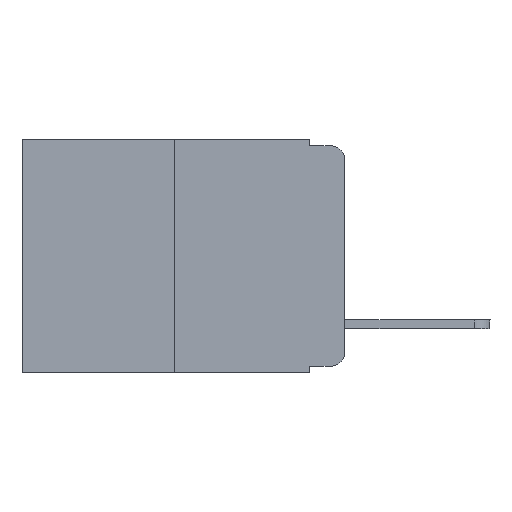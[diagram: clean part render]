
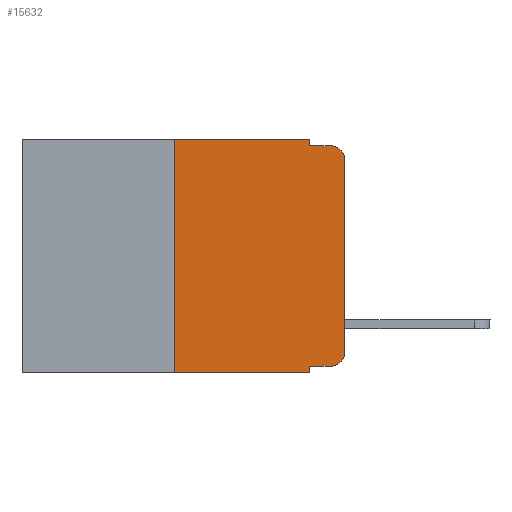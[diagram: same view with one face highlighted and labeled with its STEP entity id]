
A CAD part, left-side view. The second image highlights one B-rep face of the part: STEP entity #15632.
In plain terms, the highlighted planar face has unit normal (-1, 0, 0).
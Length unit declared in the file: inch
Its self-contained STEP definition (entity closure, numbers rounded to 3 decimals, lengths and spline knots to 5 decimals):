
#16 = VERTEX_POINT ( 'NONE', #12961 ) ;
#89 = ORIENTED_EDGE ( 'NONE', *, *, #2697, .T. ) ;
#447 = LINE ( 'NONE', #6136, #10270 ) ;
#598 = VECTOR ( 'NONE', #6425, 39.37008 ) ;
#610 = DIRECTION ( 'NONE',  ( 0., -1., 0. ) ) ;
#771 = EDGE_CURVE ( 'NONE', #15232, #12981, #5989, .T. ) ;
#961 = EDGE_CURVE ( 'NONE', #3831, #3581, #9354, .T. ) ;
#1039 = CARTESIAN_POINT ( 'NONE',  ( 0., 0.25, 0. ) ) ;
#1077 = VERTEX_POINT ( 'NONE', #1764 ) ;
#1095 = DIRECTION ( 'NONE',  ( 0., 0., 1. ) ) ;
#1254 = EDGE_CURVE ( 'NONE', #3831, #16, #9566, .T. ) ;
#1634 = DIRECTION ( 'NONE',  ( -1., 0., 0. ) ) ;
#1764 = CARTESIAN_POINT ( 'NONE',  ( 0., 0.051, 0. ) ) ;
#2280 = AXIS2_PLACEMENT_3D ( 'NONE', #14104, #15398, #8887 ) ;
#2580 = VERTEX_POINT ( 'NONE', #16187 ) ;
#2617 = ORIENTED_EDGE ( 'NONE', *, *, #11180, .T. ) ;
#2697 = EDGE_CURVE ( 'NONE', #2580, #15232, #8344, .T. ) ;
#2749 = CARTESIAN_POINT ( 'NONE',  ( 0., 0.02, -0.313 ) ) ;
#2760 = EDGE_CURVE ( 'NONE', #16, #1077, #10550, .T. ) ;
#3581 = VERTEX_POINT ( 'NONE', #16235 ) ;
#3825 = ORIENTED_EDGE ( 'NONE', *, *, #13340, .F. ) ;
#3831 = VERTEX_POINT ( 'NONE', #13111 ) ;
#3943 = DIRECTION ( 'NONE',  ( 0., 0., -1. ) ) ;
#3953 = VECTOR ( 'NONE', #12340, 39.37008 ) ;
#4468 = EDGE_LOOP ( 'NONE', ( #5801, #16324, #7175, #3825, #14455, #10237, #12030, #13215, #2617, #89 ) ) ;
#5530 = VECTOR ( 'NONE', #5571, 39.37008 ) ;
#5571 = DIRECTION ( 'NONE',  ( 0., -1., 0. ) ) ;
#5767 = EDGE_CURVE ( 'NONE', #12981, #6544, #14261, .T. ) ;
#5786 = CARTESIAN_POINT ( 'NONE',  ( 0., 0., 0. ) ) ;
#5801 = ORIENTED_EDGE ( 'NONE', *, *, #771, .T. ) ;
#5950 = VERTEX_POINT ( 'NONE', #6956 ) ;
#5989 = LINE ( 'NONE', #5786, #3953 ) ;
#6136 = CARTESIAN_POINT ( 'NONE',  ( 0., 0.051, -0.01 ) ) ;
#6361 = FACE_OUTER_BOUND ( 'NONE', #4468, .T. ) ;
#6425 = DIRECTION ( 'NONE',  ( 0., 0., -1. ) ) ;
#6487 = VECTOR ( 'NONE', #610, 39.37008 ) ;
#6544 = VERTEX_POINT ( 'NONE', #12249 ) ;
#6956 = CARTESIAN_POINT ( 'NONE',  ( 0., 0.051, -0.01 ) ) ;
#7154 = VECTOR ( 'NONE', #1095, 39.37008 ) ;
#7175 = ORIENTED_EDGE ( 'NONE', *, *, #12117, .F. ) ;
#7408 = LINE ( 'NONE', #12821, #598 ) ;
#7543 = LINE ( 'NONE', #7878, #11759 ) ;
#7745 = CARTESIAN_POINT ( 'NONE',  ( 0., 0.051, -0.333 ) ) ;
#7878 = CARTESIAN_POINT ( 'NONE',  ( 0., 0.051, 0. ) ) ;
#8079 = CARTESIAN_POINT ( 'NONE',  ( 0., 0.02, -0.03 ) ) ;
#8344 = CIRCLE ( 'NONE', #10968, 0.02 ) ;
#8750 = DIRECTION ( 'NONE',  ( 0., -1., 0. ) ) ;
#8887 = DIRECTION ( 'NONE',  ( 0., 0., -1. ) ) ;
#8998 = DIRECTION ( 'NONE',  ( -1., 0., 0. ) ) ;
#9354 = LINE ( 'NONE', #15465, #11767 ) ;
#9566 = LINE ( 'NONE', #1039, #7154 ) ;
#10237 = ORIENTED_EDGE ( 'NONE', *, *, #1254, .F. ) ;
#10270 = VECTOR ( 'NONE', #8750, 39.37008 ) ;
#10550 = LINE ( 'NONE', #15828, #5530 ) ;
#10968 = AXIS2_PLACEMENT_3D ( 'NONE', #2749, #8998, #11794 ) ;
#11180 = EDGE_CURVE ( 'NONE', #12218, #2580, #11292, .T. ) ;
#11292 = LINE ( 'NONE', #14674, #6487 ) ;
#11759 = VECTOR ( 'NONE', #3943, 39.37008 ) ;
#11767 = VECTOR ( 'NONE', #14229, 39.37008 ) ;
#11794 = DIRECTION ( 'NONE',  ( 0., 0., -1. ) ) ;
#11933 = DIRECTION ( 'NONE',  ( 0., 0., -1. ) ) ;
#12030 = ORIENTED_EDGE ( 'NONE', *, *, #961, .T. ) ;
#12117 = EDGE_CURVE ( 'NONE', #5950, #6544, #447, .T. ) ;
#12218 = VERTEX_POINT ( 'NONE', #7745 ) ;
#12249 = CARTESIAN_POINT ( 'NONE',  ( 0., 0.02, -0.01 ) ) ;
#12340 = DIRECTION ( 'NONE',  ( 0., 0., 1. ) ) ;
#12603 = AXIS2_PLACEMENT_3D ( 'NONE', #8079, #1634, #11933 ) ;
#12821 = CARTESIAN_POINT ( 'NONE',  ( 0., 0.051, 0. ) ) ;
#12961 = CARTESIAN_POINT ( 'NONE',  ( 0., 0.25, 0. ) ) ;
#12981 = VERTEX_POINT ( 'NONE', #16070 ) ;
#13111 = CARTESIAN_POINT ( 'NONE',  ( 0., 0.25, -0.343 ) ) ;
#13215 = ORIENTED_EDGE ( 'NONE', *, *, #15668, .F. ) ;
#13340 = EDGE_CURVE ( 'NONE', #1077, #5950, #7408, .T. ) ;
#14104 = CARTESIAN_POINT ( 'NONE',  ( 0., 0.473, 0. ) ) ;
#14229 = DIRECTION ( 'NONE',  ( 0., -1., 0. ) ) ;
#14261 = CIRCLE ( 'NONE', #12603, 0.02 ) ;
#14455 = ORIENTED_EDGE ( 'NONE', *, *, #2760, .F. ) ;
#14674 = CARTESIAN_POINT ( 'NONE',  ( 0., 0.051, -0.333 ) ) ;
#15232 = VERTEX_POINT ( 'NONE', #15687 ) ;
#15398 = DIRECTION ( 'NONE',  ( 1., 0., 0. ) ) ;
#15465 = CARTESIAN_POINT ( 'NONE',  ( 0., 0.473, -0.343 ) ) ;
#15632 = ADVANCED_FACE ( 'NONE', ( #6361 ), #16555, .F. ) ;
#15668 = EDGE_CURVE ( 'NONE', #12218, #3581, #7543, .T. ) ;
#15687 = CARTESIAN_POINT ( 'NONE',  ( 0., 0., -0.313 ) ) ;
#15828 = CARTESIAN_POINT ( 'NONE',  ( 0., 0.473, 0. ) ) ;
#16070 = CARTESIAN_POINT ( 'NONE',  ( 0., 0., -0.03 ) ) ;
#16187 = CARTESIAN_POINT ( 'NONE',  ( 0., 0.02, -0.333 ) ) ;
#16235 = CARTESIAN_POINT ( 'NONE',  ( 0., 0.051, -0.343 ) ) ;
#16324 = ORIENTED_EDGE ( 'NONE', *, *, #5767, .T. ) ;
#16555 = PLANE ( 'NONE',  #2280 ) ;
